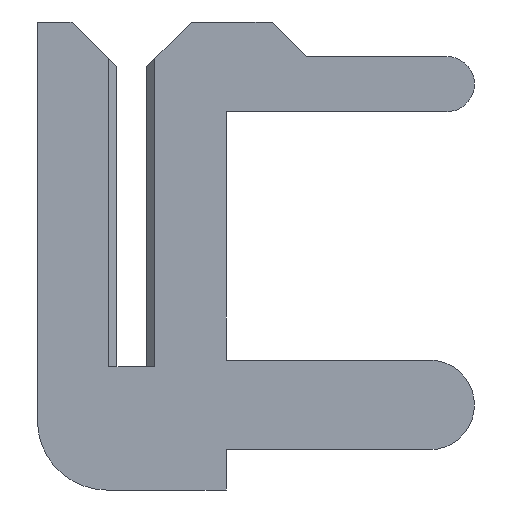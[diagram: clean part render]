
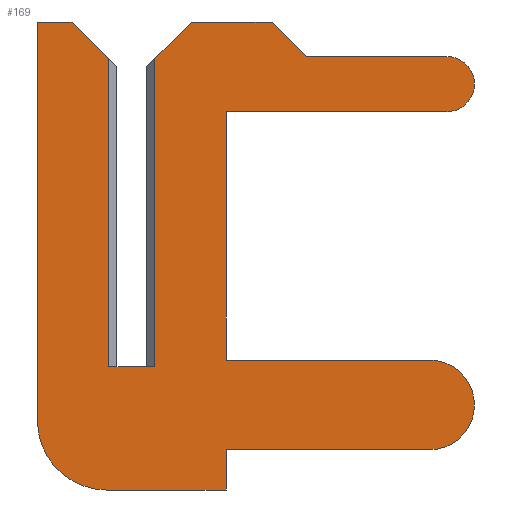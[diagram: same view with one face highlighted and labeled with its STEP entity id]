
A CAD part, left-side view. The second image highlights one B-rep face of the part: STEP entity #169.
In plain terms, the highlighted planar face has unit normal (-1, 0, 0).
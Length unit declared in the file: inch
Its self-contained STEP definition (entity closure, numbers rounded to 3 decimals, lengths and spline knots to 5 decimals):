
#4 = LINE ( 'NONE', #917, #1375 ) ;
#6 = EDGE_CURVE ( 'NONE', #895, #1109, #4, .T. ) ;
#11 = CARTESIAN_POINT ( 'NONE',  ( -0.01, 0.01, -0.0235 ) ) ;
#12 = ORIENTED_EDGE ( 'NONE', *, *, #372, .F. ) ;
#32 = CARTESIAN_POINT ( 'NONE',  ( -0.01, 0.01, 0. ) ) ;
#73 = CARTESIAN_POINT ( 'NONE',  ( -0.01, -0.01, 0.15 ) ) ;
#83 = CARTESIAN_POINT ( 'NONE',  ( -0.01, 0.01, 0.134 ) ) ;
#92 = CARTESIAN_POINT ( 'NONE',  ( -0.01, -0.0065, 0.1305 ) ) ;
#110 = LINE ( 'NONE', #1303, #488 ) ;
#117 = DIRECTION ( 'NONE',  ( 0., -0.707, -0.707 ) ) ;
#133 = CARTESIAN_POINT ( 'NONE',  ( -0.01, 0.026, 0.15 ) ) ;
#141 = VERTEX_POINT ( 'NONE', #581 ) ;
#147 = DIRECTION ( 'NONE',  ( 1., 0., 0. ) ) ;
#169 = ADVANCED_FACE ( 'NONE', ( #858 ), #1376, .T. ) ;
#188 = CARTESIAN_POINT ( 'NONE',  ( -0.01, -0.137, 0.123 ) ) ;
#191 = DIRECTION ( 'NONE',  ( -1., 0., 0. ) ) ;
#199 = ORIENTED_EDGE ( 'NONE', *, *, #6, .F. ) ;
#207 = CARTESIAN_POINT ( 'NONE',  ( -0.01, 0.041, 0.15 ) ) ;
#224 = VERTEX_POINT ( 'NONE', #83 ) ;
#228 = AXIS2_PLACEMENT_3D ( 'NONE', #1159, #953, #416 ) ;
#229 = EDGE_LOOP ( 'NONE', ( #440, #802, #278, #336, #475, #1130, #199, #672, #512, #12, #1058, #720, #951, #735, #775, #697, #850, #1321, #528 ) ) ;
#237 = DIRECTION ( 'NONE',  ( 0., -1., 0. ) ) ;
#239 = VERTEX_POINT ( 'NONE', #1160 ) ;
#245 = EDGE_CURVE ( 'NONE', #1165, #141, #753, .T. ) ;
#247 = CARTESIAN_POINT ( 'NONE',  ( -0.01, -0.137, 0.111 ) ) ;
#248 = EDGE_CURVE ( 'NONE', #1348, #954, #1293, .T. ) ;
#258 = DIRECTION ( 'NONE',  ( 0., 0., 1. ) ) ;
#259 = VERTEX_POINT ( 'NONE', #1368 ) ;
#275 = VECTOR ( 'NONE', #667, 39.37008 ) ;
#278 = ORIENTED_EDGE ( 'NONE', *, *, #607, .F. ) ;
#297 = CARTESIAN_POINT ( 'NONE',  ( -0.01, 0.041, -0.0235 ) ) ;
#298 = LINE ( 'NONE', #894, #275 ) ;
#300 = CARTESIAN_POINT ( 'NONE',  ( -0.01, -0.041, -0.036 ) ) ;
#309 = LINE ( 'NONE', #1179, #1127 ) ;
#313 = VECTOR ( 'NONE', #873, 39.37008 ) ;
#321 = VERTEX_POINT ( 'NONE', #606 ) ;
#336 = ORIENTED_EDGE ( 'NONE', *, *, #1189, .T. ) ;
#348 = CARTESIAN_POINT ( 'NONE',  ( -0.01, 0.026, 0.15 ) ) ;
#350 = CIRCLE ( 'NONE', #1072, 0.012 ) ;
#367 = CARTESIAN_POINT ( 'NONE',  ( -0.01, -0.137, 0.135 ) ) ;
#372 = EDGE_CURVE ( 'NONE', #141, #1348, #298, .T. ) ;
#385 = CARTESIAN_POINT ( 'NONE',  ( -0.01, 0.011, -0.0535 ) ) ;
#404 = EDGE_CURVE ( 'NONE', #884, #239, #517, .T. ) ;
#412 = CIRCLE ( 'NONE', #674, 0.0195 ) ;
#413 = CARTESIAN_POINT ( 'NONE',  ( -0.01, -0.1295, -0.036 ) ) ;
#416 = DIRECTION ( 'NONE',  ( 0., 0., 1. ) ) ;
#427 = EDGE_CURVE ( 'NONE', #1109, #626, #1183, .T. ) ;
#437 = EDGE_CURVE ( 'NONE', #650, #717, #110, .T. ) ;
#440 = ORIENTED_EDGE ( 'NONE', *, *, #879, .F. ) ;
#443 = VECTOR ( 'NONE', #927, 39.37008 ) ;
#445 = VERTEX_POINT ( 'NONE', #562 ) ;
#452 = VERTEX_POINT ( 'NONE', #978 ) ;
#454 = EDGE_CURVE ( 'NONE', #455, #321, #889, .T. ) ;
#455 = VERTEX_POINT ( 'NONE', #552 ) ;
#475 = ORIENTED_EDGE ( 'NONE', *, *, #1067, .F. ) ;
#488 = VECTOR ( 'NONE', #237, 39.37008 ) ;
#512 = ORIENTED_EDGE ( 'NONE', *, *, #248, .F. ) ;
#517 = LINE ( 'NONE', #1110, #1059 ) ;
#528 = ORIENTED_EDGE ( 'NONE', *, *, #404, .F. ) ;
#531 = EDGE_CURVE ( 'NONE', #445, #455, #968, .T. ) ;
#532 = LINE ( 'NONE', #958, #854 ) ;
#550 = VERTEX_POINT ( 'NONE', #247 ) ;
#552 = CARTESIAN_POINT ( 'NONE',  ( -0.01, -0.041, 0.003 ) ) ;
#562 = CARTESIAN_POINT ( 'NONE',  ( -0.01, -0.041, 0.111 ) ) ;
#563 = CARTESIAN_POINT ( 'NONE',  ( -0.01, -0.041, 0.003 ) ) ;
#581 = CARTESIAN_POINT ( 'NONE',  ( -0.01, -0.041, -0.036 ) ) ;
#606 = CARTESIAN_POINT ( 'NONE',  ( -0.01, -0.1295, 0.003 ) ) ;
#607 = EDGE_CURVE ( 'NONE', #1340, #259, #885, .T. ) ;
#626 = VERTEX_POINT ( 'NONE', #133 ) ;
#650 = VERTEX_POINT ( 'NONE', #1237 ) ;
#654 = DIRECTION ( 'NONE',  ( 0., 0., -1. ) ) ;
#657 = CARTESIAN_POINT ( 'NONE',  ( -0.01, -0.1295, 0.003 ) ) ;
#662 = DIRECTION ( 'NONE',  ( 0., -1., 0. ) ) ;
#663 = LINE ( 'NONE', #92, #443 ) ;
#667 = DIRECTION ( 'NONE',  ( 0., 0., -1. ) ) ;
#672 = ORIENTED_EDGE ( 'NONE', *, *, #1122, .F. ) ;
#674 = AXIS2_PLACEMENT_3D ( 'NONE', #1331, #147, #1243 ) ;
#696 = EDGE_CURVE ( 'NONE', #321, #1165, #412, .T. ) ;
#697 = ORIENTED_EDGE ( 'NONE', *, *, #1326, .F. ) ;
#706 = VECTOR ( 'NONE', #980, 39.37008 ) ;
#709 = VECTOR ( 'NONE', #1373, 39.37008 ) ;
#717 = VERTEX_POINT ( 'NONE', #367 ) ;
#719 = CARTESIAN_POINT ( 'NONE',  ( -0.01, -0.026, 0.15 ) ) ;
#720 = ORIENTED_EDGE ( 'NONE', *, *, #696, .F. ) ;
#724 = LINE ( 'NONE', #896, #955 ) ;
#735 = ORIENTED_EDGE ( 'NONE', *, *, #531, .F. ) ;
#753 = LINE ( 'NONE', #300, #709 ) ;
#758 = EDGE_CURVE ( 'NONE', #452, #259, #1005, .T. ) ;
#764 = CARTESIAN_POINT ( 'NONE',  ( -0.01, 0.0065, 0. ) ) ;
#765 = VECTOR ( 'NONE', #1117, 39.37008 ) ;
#775 = ORIENTED_EDGE ( 'NONE', *, *, #1023, .F. ) ;
#802 = ORIENTED_EDGE ( 'NONE', *, *, #758, .T. ) ;
#816 = DIRECTION ( 'NONE',  ( 1., 0., 0. ) ) ;
#840 = EDGE_CURVE ( 'NONE', #239, #650, #724, .T. ) ;
#850 = ORIENTED_EDGE ( 'NONE', *, *, #437, .F. ) ;
#854 = VECTOR ( 'NONE', #117, 39.37008 ) ;
#858 = FACE_OUTER_BOUND ( 'NONE', #229, .T. ) ;
#873 = DIRECTION ( 'NONE',  ( 0., -1., 0. ) ) ;
#879 = EDGE_CURVE ( 'NONE', #452, #884, #663, .T. ) ;
#884 = VERTEX_POINT ( 'NONE', #719 ) ;
#885 = LINE ( 'NONE', #764, #706 ) ;
#889 = LINE ( 'NONE', #657, #1107 ) ;
#894 = CARTESIAN_POINT ( 'NONE',  ( -0.01, -0.041, -0.0535 ) ) ;
#895 = VERTEX_POINT ( 'NONE', #297 ) ;
#896 = CARTESIAN_POINT ( 'NONE',  ( -0.01, -0.076, 0.135 ) ) ;
#917 = CARTESIAN_POINT ( 'NONE',  ( -0.01, 0.041, 0.15 ) ) ;
#923 = LINE ( 'NONE', #11, #1211 ) ;
#927 = DIRECTION ( 'NONE',  ( 0., -0.707, 0.707 ) ) ;
#931 = DIRECTION ( 'NONE',  ( 0., 0., 1. ) ) ;
#934 = CARTESIAN_POINT ( 'NONE',  ( -0.01, 0.011, -0.0535 ) ) ;
#951 = ORIENTED_EDGE ( 'NONE', *, *, #454, .F. ) ;
#953 = DIRECTION ( 'NONE',  ( 1., 0., 0. ) ) ;
#954 = VERTEX_POINT ( 'NONE', #934 ) ;
#955 = VECTOR ( 'NONE', #1123, 39.37008 ) ;
#957 = VECTOR ( 'NONE', #1148, 39.37008 ) ;
#958 = CARTESIAN_POINT ( 'NONE',  ( -0.01, 0.0065, 0.1305 ) ) ;
#968 = LINE ( 'NONE', #563, #1276 ) ;
#978 = CARTESIAN_POINT ( 'NONE',  ( -0.01, -0.01, 0.134 ) ) ;
#980 = DIRECTION ( 'NONE',  ( 0., -1., 0. ) ) ;
#1005 = LINE ( 'NONE', #73, #765 ) ;
#1023 = EDGE_CURVE ( 'NONE', #550, #445, #309, .T. ) ;
#1058 = ORIENTED_EDGE ( 'NONE', *, *, #245, .F. ) ;
#1059 = VECTOR ( 'NONE', #1095, 39.37008 ) ;
#1067 = EDGE_CURVE ( 'NONE', #626, #224, #532, .T. ) ;
#1072 = AXIS2_PLACEMENT_3D ( 'NONE', #188, #816, #1300 ) ;
#1095 = DIRECTION ( 'NONE',  ( 0., -1., 0. ) ) ;
#1099 = CARTESIAN_POINT ( 'NONE',  ( -0.01, -0.041, -0.0535 ) ) ;
#1107 = VECTOR ( 'NONE', #662, 39.37008 ) ;
#1109 = VERTEX_POINT ( 'NONE', #207 ) ;
#1110 = CARTESIAN_POINT ( 'NONE',  ( -0.01, -0.026, 0.15 ) ) ;
#1117 = DIRECTION ( 'NONE',  ( 0., 0., -1. ) ) ;
#1122 = EDGE_CURVE ( 'NONE', #954, #895, #1278, .T. ) ;
#1123 = DIRECTION ( 'NONE',  ( 0., -0.707, -0.707 ) ) ;
#1127 = VECTOR ( 'NONE', #1281, 39.37008 ) ;
#1130 = ORIENTED_EDGE ( 'NONE', *, *, #427, .F. ) ;
#1148 = DIRECTION ( 'NONE',  ( 0., 1., 0. ) ) ;
#1159 = CARTESIAN_POINT ( 'NONE',  ( -0.01, 0.011, -0.0235 ) ) ;
#1160 = CARTESIAN_POINT ( 'NONE',  ( -0.01, -0.061, 0.15 ) ) ;
#1165 = VERTEX_POINT ( 'NONE', #413 ) ;
#1179 = CARTESIAN_POINT ( 'NONE',  ( -0.01, -0.041, 0.111 ) ) ;
#1183 = LINE ( 'NONE', #348, #313 ) ;
#1189 = EDGE_CURVE ( 'NONE', #1340, #224, #923, .T. ) ;
#1211 = VECTOR ( 'NONE', #1289, 39.37008 ) ;
#1237 = CARTESIAN_POINT ( 'NONE',  ( -0.01, -0.076, 0.135 ) ) ;
#1243 = DIRECTION ( 'NONE',  ( 0., 0., 1. ) ) ;
#1252 = CARTESIAN_POINT ( 'NONE',  ( -0.01, 0.011, -0.0235 ) ) ;
#1276 = VECTOR ( 'NONE', #654, 39.37008 ) ;
#1278 = CIRCLE ( 'NONE', #228, 0.03 ) ;
#1281 = DIRECTION ( 'NONE',  ( 0., 1., 0. ) ) ;
#1289 = DIRECTION ( 'NONE',  ( 0., 0., 1. ) ) ;
#1293 = LINE ( 'NONE', #385, #957 ) ;
#1300 = DIRECTION ( 'NONE',  ( 0., 0., 1. ) ) ;
#1303 = CARTESIAN_POINT ( 'NONE',  ( -0.01, -0.137, 0.135 ) ) ;
#1321 = ORIENTED_EDGE ( 'NONE', *, *, #840, .F. ) ;
#1326 = EDGE_CURVE ( 'NONE', #717, #550, #350, .T. ) ;
#1331 = CARTESIAN_POINT ( 'NONE',  ( -0.01, -0.1295, -0.0165 ) ) ;
#1340 = VERTEX_POINT ( 'NONE', #32 ) ;
#1344 = AXIS2_PLACEMENT_3D ( 'NONE', #1252, #191, #931 ) ;
#1348 = VERTEX_POINT ( 'NONE', #1099 ) ;
#1368 = CARTESIAN_POINT ( 'NONE',  ( -0.01, -0.01, 0. ) ) ;
#1373 = DIRECTION ( 'NONE',  ( 0., 1., 0. ) ) ;
#1375 = VECTOR ( 'NONE', #258, 39.37008 ) ;
#1376 = PLANE ( 'NONE',  #1344 ) ;
